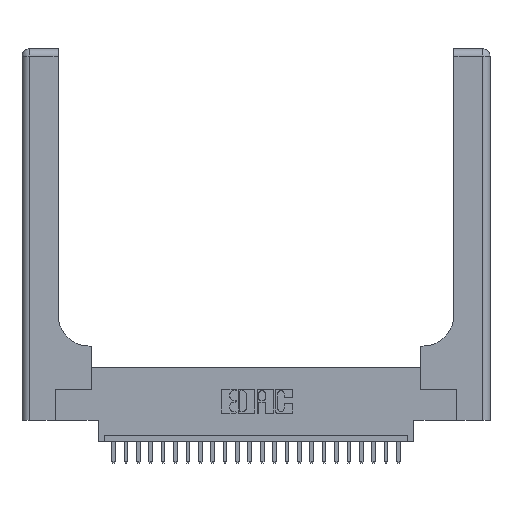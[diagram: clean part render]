
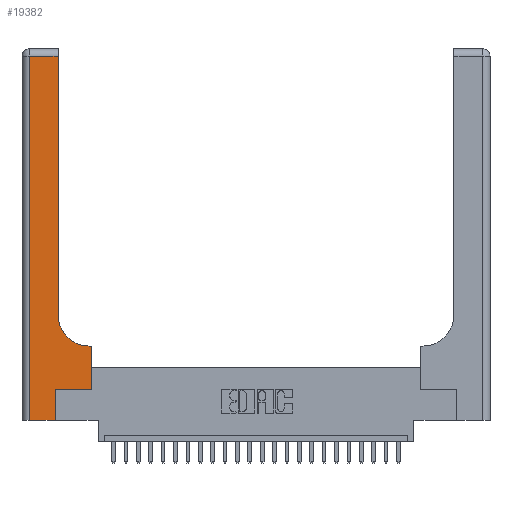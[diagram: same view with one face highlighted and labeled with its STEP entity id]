
A CAD part, top view. The second image highlights one B-rep face of the part: STEP entity #19382.
In plain terms, the highlighted planar face has unit normal (0, 0, 1).
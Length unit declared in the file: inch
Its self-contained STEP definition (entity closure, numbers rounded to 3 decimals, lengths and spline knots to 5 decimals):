
#22 = EDGE_CURVE ( 'NONE', #10821, #12915, #10415, .T. ) ;
#27 = CARTESIAN_POINT ( 'NONE',  ( 0.269, 0.25, 0.37 ) ) ;
#240 = CARTESIAN_POINT ( 'NONE',  ( 0.2915, 0.85, 0.37 ) ) ;
#520 = VECTOR ( 'NONE', #16933, 39.37008 ) ;
#847 = VECTOR ( 'NONE', #11407, 39.37008 ) ;
#1507 = DIRECTION ( 'NONE',  ( 0., 0., -1. ) ) ;
#2262 = FACE_OUTER_BOUND ( 'NONE', #18681, .T. ) ;
#2462 = PLANE ( 'NONE',  #17873 ) ;
#2760 = VECTOR ( 'NONE', #5846, 39.37008 ) ;
#2825 = CARTESIAN_POINT ( 'NONE',  ( 0.5415, 0.85, 0.37 ) ) ;
#2934 = CARTESIAN_POINT ( 'NONE',  ( 0., 2.94, 0.37 ) ) ;
#3044 = LINE ( 'NONE', #25189, #9357 ) ;
#3524 = EDGE_CURVE ( 'NONE', #20379, #23088, #20288, .T. ) ;
#3752 = EDGE_CURVE ( 'NONE', #13357, #19452, #24642, .T. ) ;
#4020 = ORIENTED_EDGE ( 'NONE', *, *, #4589, .T. ) ;
#4037 = VECTOR ( 'NONE', #7393, 39.37008 ) ;
#4589 = EDGE_CURVE ( 'NONE', #12915, #20603, #8318, .T. ) ;
#5734 = VERTEX_POINT ( 'NONE', #18157 ) ;
#5846 = DIRECTION ( 'NONE',  ( 0., -1., 0. ) ) ;
#5941 = VECTOR ( 'NONE', #17721, 39.37008 ) ;
#6159 = ORIENTED_EDGE ( 'NONE', *, *, #3524, .T. ) ;
#6251 = EDGE_CURVE ( 'NONE', #23088, #15015, #9547, .T. ) ;
#6645 = AXIS2_PLACEMENT_3D ( 'NONE', #2825, #1507, #19930 ) ;
#7267 = CARTESIAN_POINT ( 'NONE',  ( 0.2915, 0.6, 0.37 ) ) ;
#7393 = DIRECTION ( 'NONE',  ( 0., 1., 0. ) ) ;
#8318 = LINE ( 'NONE', #11122, #14581 ) ;
#9306 = CARTESIAN_POINT ( 'NONE',  ( 0.06, 0., 0.37 ) ) ;
#9357 = VECTOR ( 'NONE', #15752, 39.37008 ) ;
#9390 = LINE ( 'NONE', #12124, #5941 ) ;
#9547 = CIRCLE ( 'NONE', #6645, 0.25 ) ;
#10415 = LINE ( 'NONE', #18284, #12933 ) ;
#10821 = VERTEX_POINT ( 'NONE', #9306 ) ;
#11122 = CARTESIAN_POINT ( 'NONE',  ( 0.269, 0., 0.37 ) ) ;
#11310 = ORIENTED_EDGE ( 'NONE', *, *, #13451, .T. ) ;
#11407 = DIRECTION ( 'NONE',  ( -1., 0., 0. ) ) ;
#11718 = CARTESIAN_POINT ( 'NONE',  ( 0.06, 3., 0.37 ) ) ;
#11971 = CARTESIAN_POINT ( 'NONE',  ( 0.269, 0., 0.37 ) ) ;
#12124 = CARTESIAN_POINT ( 'NONE',  ( 0.2915, 3., 0.37 ) ) ;
#12737 = ORIENTED_EDGE ( 'NONE', *, *, #3752, .T. ) ;
#12844 = DIRECTION ( 'NONE',  ( 1., 0., 0. ) ) ;
#12861 = EDGE_CURVE ( 'NONE', #19452, #10821, #19412, .T. ) ;
#12915 = VERTEX_POINT ( 'NONE', #11971 ) ;
#12933 = VECTOR ( 'NONE', #12844, 39.37008 ) ;
#13357 = VERTEX_POINT ( 'NONE', #17238 ) ;
#13451 = EDGE_CURVE ( 'NONE', #20603, #5734, #3044, .T. ) ;
#13543 = CARTESIAN_POINT ( 'NONE',  ( 0.5585, 0.6, 0.37 ) ) ;
#14581 = VECTOR ( 'NONE', #25233, 39.37008 ) ;
#14988 = LINE ( 'NONE', #19292, #4037 ) ;
#15015 = VERTEX_POINT ( 'NONE', #240 ) ;
#15752 = DIRECTION ( 'NONE',  ( 1., 0., 0. ) ) ;
#16101 = ORIENTED_EDGE ( 'NONE', *, *, #6251, .T. ) ;
#16538 = EDGE_CURVE ( 'NONE', #15015, #13357, #9390, .T. ) ;
#16933 = DIRECTION ( 'NONE',  ( -1., 0., 0. ) ) ;
#17086 = ORIENTED_EDGE ( 'NONE', *, *, #22695, .T. ) ;
#17238 = CARTESIAN_POINT ( 'NONE',  ( 0.2915, 2.94, 0.37 ) ) ;
#17721 = DIRECTION ( 'NONE',  ( 0., 1., 0. ) ) ;
#17873 = AXIS2_PLACEMENT_3D ( 'NONE', #20260, #22360, #18508 ) ;
#18157 = CARTESIAN_POINT ( 'NONE',  ( 0.5585, 0.25, 0.37 ) ) ;
#18284 = CARTESIAN_POINT ( 'NONE',  ( 0., 0., 0.37 ) ) ;
#18508 = DIRECTION ( 'NONE',  ( -1., 0., 0. ) ) ;
#18681 = EDGE_LOOP ( 'NONE', ( #25790, #12737, #22514, #20825, #4020, #11310, #17086, #6159, #16101 ) ) ;
#18684 = CARTESIAN_POINT ( 'NONE',  ( 0.06, 2.94, 0.37 ) ) ;
#19292 = CARTESIAN_POINT ( 'NONE',  ( 0.5585, 0.25, 0.37 ) ) ;
#19364 = CARTESIAN_POINT ( 'NONE',  ( 0.5415, 0.6, 0.37 ) ) ;
#19382 = ADVANCED_FACE ( 'NONE', ( #2262 ), #2462, .F. ) ;
#19412 = LINE ( 'NONE', #11718, #2760 ) ;
#19452 = VERTEX_POINT ( 'NONE', #18684 ) ;
#19930 = DIRECTION ( 'NONE',  ( 1., 0., 0. ) ) ;
#20260 = CARTESIAN_POINT ( 'NONE',  ( 0., 3., 0.37 ) ) ;
#20288 = LINE ( 'NONE', #7267, #847 ) ;
#20379 = VERTEX_POINT ( 'NONE', #13543 ) ;
#20603 = VERTEX_POINT ( 'NONE', #27 ) ;
#20825 = ORIENTED_EDGE ( 'NONE', *, *, #22, .T. ) ;
#22360 = DIRECTION ( 'NONE',  ( 0., 0., -1. ) ) ;
#22514 = ORIENTED_EDGE ( 'NONE', *, *, #12861, .T. ) ;
#22695 = EDGE_CURVE ( 'NONE', #5734, #20379, #14988, .T. ) ;
#23088 = VERTEX_POINT ( 'NONE', #19364 ) ;
#24642 = LINE ( 'NONE', #2934, #520 ) ;
#25189 = CARTESIAN_POINT ( 'NONE',  ( 0.269, 0.25, 0.37 ) ) ;
#25233 = DIRECTION ( 'NONE',  ( 0., 1., 0. ) ) ;
#25790 = ORIENTED_EDGE ( 'NONE', *, *, #16538, .T. ) ;
